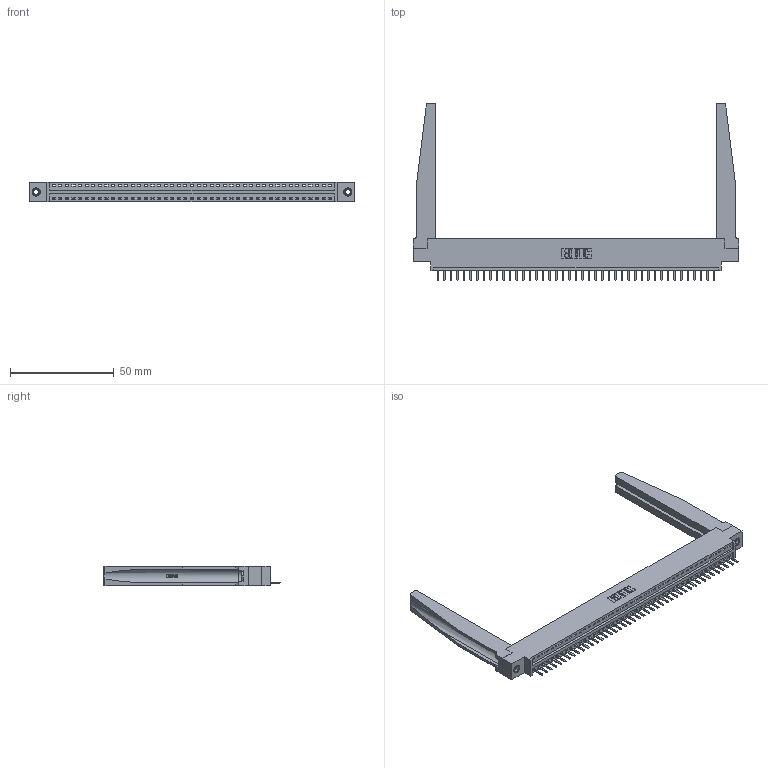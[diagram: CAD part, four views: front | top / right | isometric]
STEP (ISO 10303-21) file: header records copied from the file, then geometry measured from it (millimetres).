
FILE_DESCRIPTION (( 'STEP AP203' ), '1' );
FILE_NAME ('346-043-520-678.STEP', '2022-05-09T15:22:51', ( '' ), ( '' ), 'SwSTEP 2.0', 'SolidWorks 2020', '' );
FILE_SCHEMA (( 'CONFIG_CONTROL_DESIGN' ));
Length unit declared in the file: inch
Products named in the file (5): 346 Part_0.170 Offset - 0.156 Dia-TH; 346-043-520-678; 346-220-078_345-220-078; 345-292-001_345-293-120; 345-250-001_345-250-001-102
Assembly tree (48 placements, depth 2):
  346-043-520-678
    346 Part_0.170 Offset - 0.156 Dia-TH
    345-292-001_345-293-120  x43
    346-220-078_345-220-078  x2
    345-250-001_345-250-001-102  x2
Bounding box: 157.1 x 85.29 x 9.4 mm (x, y, z)
Volume: 21657.2 mm3; surface area: 24764.1 mm2
Topology: 48 solids, 48 shells, 3040 faces, 8897 edges, 5806 vertices
Faces by surface type: plane 2042, cylinder 946, bspline 36, cone 12, torus 4
Entity records: 31962 total; most frequent: CARTESIAN_POINT 6406, ORIENTED_EDGE 5258, DIRECTION 4621, EDGE_CURVE 2629, VECTOR 2227, LINE 2227, VERTEX_POINT 1744, AXIS2_PLACEMENT_3D 1197
